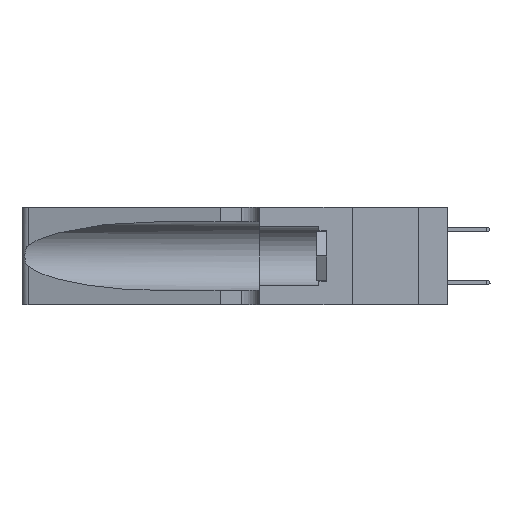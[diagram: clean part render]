
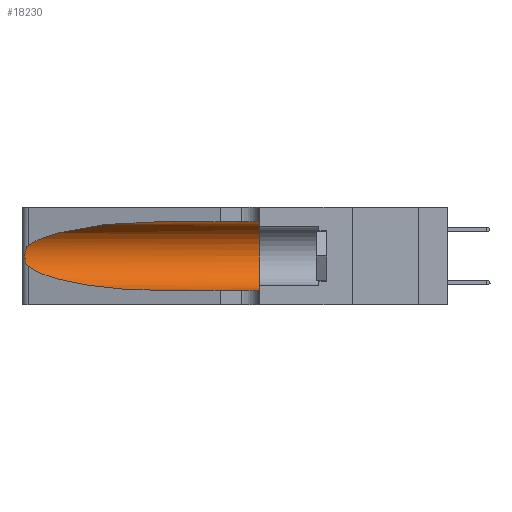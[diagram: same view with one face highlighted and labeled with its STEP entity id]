
A CAD part, left-side view. The second image highlights one B-rep face of the part: STEP entity #18230.
In plain terms, the highlighted cylindrical face has radius 3.308 mm (diameter 6.617 mm), a partial arc.
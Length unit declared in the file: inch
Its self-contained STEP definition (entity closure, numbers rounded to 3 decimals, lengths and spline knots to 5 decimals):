
#116 = CYLINDRICAL_SURFACE ( 'NONE', #184, 0.13025 ) ;
#184 = AXIS2_PLACEMENT_3D ( 'NONE', #6287, #4804, #3299 ) ;
#208 = ORIENTED_EDGE ( 'NONE', *, *, #14367, .T. ) ;
#456 = CARTESIAN_POINT ( 'NONE',  ( 0.25639, 1.23184, 0.21858 ) ) ;
#737 = VECTOR ( 'NONE', #8230, 39.37008 ) ;
#919 = DIRECTION ( 'NONE',  ( 0., -1., 0. ) ) ;
#948 = DIRECTION ( 'NONE',  ( 0., 0., 1. ) ) ;
#1972 = CARTESIAN_POINT ( 'NONE',  ( 0.25854, 1.2359, 0.20912 ) ) ;
#2413 = CARTESIAN_POINT ( 'NONE',  ( 0.1305, 0.72297, 0.31525 ) ) ;
#2427 = CARTESIAN_POINT ( 'NONE',  ( 0.1305, 1.61858, 0.05475 ) ) ;
#2509 =( BOUNDED_CURVE ( )  B_SPLINE_CURVE ( 3, ( #2413, #14236, #17169, #8345 ),
 .UNSPECIFIED., .F., .T. ) 
 B_SPLINE_CURVE_WITH_KNOTS ( ( 4, 4 ),
 ( 1.5708, 2.84003 ),
 .UNSPECIFIED. ) 
 CURVE ( )  GEOMETRIC_REPRESENTATION_ITEM ( )  RATIONAL_B_SPLINE_CURVE ( ( 1., 0.87, 0.87, 1. ) ) 
 REPRESENTATION_ITEM ( '' )  );
#2665 = VERTEX_POINT ( 'NONE', #16208 ) ;
#3154 = EDGE_CURVE ( 'NONE', #6895, #15905, #10402, .T. ) ;
#3299 = DIRECTION ( 'NONE',  ( 0., 0., -1. ) ) ;
#3495 = CARTESIAN_POINT ( 'NONE',  ( 0.26075, 1.23896, 0.19203 ) ) ;
#4143 = FACE_OUTER_BOUND ( 'NONE', #4858, .T. ) ;
#4450 = VERTEX_POINT ( 'NONE', #17107 ) ;
#4804 = DIRECTION ( 'NONE',  ( 0., -1., 0. ) ) ;
#4858 = EDGE_LOOP ( 'NONE', ( #208, #18872, #9476, #4998, #5190, #18024 ) ) ;
#4991 = CARTESIAN_POINT ( 'NONE',  ( 0.26017, 1.23833, 0.17102 ) ) ;
#4998 = ORIENTED_EDGE ( 'NONE', *, *, #18517, .T. ) ;
#5190 = ORIENTED_EDGE ( 'NONE', *, *, #16940, .F. ) ;
#5484 = CARTESIAN_POINT ( 'NONE',  ( 0.2373, 1.15595, 0.08982 ) ) ;
#5829 = CARTESIAN_POINT ( 'NONE',  ( 0.1305, 0.72297, 0.05475 ) ) ;
#6287 = CARTESIAN_POINT ( 'NONE',  ( 0.1305, 1.61858, 0.185 ) ) ;
#6468 = CARTESIAN_POINT ( 'NONE',  ( 0.25789, 1.23486, 0.15765 ) ) ;
#6856 = CARTESIAN_POINT ( 'NONE',  ( 0.25487, 1.22718, 0.14631 ) ) ;
#6864 = EDGE_CURVE ( 'NONE', #9983, #4450, #8609, .T. ) ;
#6874 = VECTOR ( 'NONE', #919, 39.37008 ) ;
#6895 = VERTEX_POINT ( 'NONE', #6856 ) ;
#7844 = CARTESIAN_POINT ( 'NONE',  ( 0.25487, 1.22718, 0.22369 ) ) ;
#7904 = CARTESIAN_POINT ( 'NONE',  ( 0.25555, 1.22993, 0.14849 ) ) ;
#8162 = CARTESIAN_POINT ( 'NONE',  ( 0.1305, 1.61858, 0.31525 ) ) ;
#8230 = DIRECTION ( 'NONE',  ( 0., -1., 0. ) ) ;
#8345 = CARTESIAN_POINT ( 'NONE',  ( 0.25487, 1.22718, 0.22369 ) ) ;
#8609 = LINE ( 'NONE', #8162, #737 ) ;
#9325 = CARTESIAN_POINT ( 'NONE',  ( 0.25555, 1.22994, 0.2215 ) ) ;
#9476 = ORIENTED_EDGE ( 'NONE', *, *, #3154, .T. ) ;
#9815 = DIRECTION ( 'NONE',  ( 0., 1., 0. ) ) ;
#9876 = CARTESIAN_POINT ( 'NONE',  ( 0.18966, 0.96281, 0.05475 ) ) ;
#9983 = VERTEX_POINT ( 'NONE', #12417 ) ;
#10402 =( BOUNDED_CURVE ( )  B_SPLINE_CURVE ( 3, ( #12870, #5484, #9876, #14346 ),
 .UNSPECIFIED., .F., .F. ) 
 B_SPLINE_CURVE_WITH_KNOTS ( ( 4, 4 ),
 ( 3.44316, 4.71239 ),
 .UNSPECIFIED. ) 
 CURVE ( )  GEOMETRIC_REPRESENTATION_ITEM ( )  RATIONAL_B_SPLINE_CURVE ( ( 1., 0.87, 0.87, 1. ) ) 
 REPRESENTATION_ITEM ( '' )  );
#10830 = CARTESIAN_POINT ( 'NONE',  ( 0.25787, 1.23484, 0.2124 ) ) ;
#11061 = CARTESIAN_POINT ( 'NONE',  ( 0.25487, 1.22718, 0.22369 ) ) ;
#11122 = EDGE_CURVE ( 'NONE', #11437, #6895, #16810, .T. ) ;
#11437 = VERTEX_POINT ( 'NONE', #11061 ) ;
#12302 = CARTESIAN_POINT ( 'NONE',  ( 0.26018, 1.23835, 0.19895 ) ) ;
#12417 = CARTESIAN_POINT ( 'NONE',  ( 0.1305, 0.72297, 0.31525 ) ) ;
#12870 = CARTESIAN_POINT ( 'NONE',  ( 0.25487, 1.22718, 0.14631 ) ) ;
#13787 = CARTESIAN_POINT ( 'NONE',  ( 0.26075, 1.23896, 0.178 ) ) ;
#14236 = CARTESIAN_POINT ( 'NONE',  ( 0.18966, 0.96281, 0.31525 ) ) ;
#14346 = CARTESIAN_POINT ( 'NONE',  ( 0.1305, 0.72297, 0.05475 ) ) ;
#14367 = EDGE_CURVE ( 'NONE', #9983, #11437, #2509, .T. ) ;
#15286 = CARTESIAN_POINT ( 'NONE',  ( 0.25856, 1.23593, 0.16098 ) ) ;
#15905 = VERTEX_POINT ( 'NONE', #5829 ) ;
#16208 = CARTESIAN_POINT ( 'NONE',  ( 0.1305, 0.35, 0.05475 ) ) ;
#16742 = CARTESIAN_POINT ( 'NONE',  ( 0.25639, 1.23186, 0.15144 ) ) ;
#16810 = B_SPLINE_CURVE_WITH_KNOTS ( 'NONE', 3,
 ( #7844, #9325, #456, #10830, #1972, #12302, #3495, #13787, #4991, #15286, #6468, #16742, #7904, #18205 ),
 .UNSPECIFIED., .F., .F.,
 ( 4, 2, 2, 2, 2, 2, 4 ),
 ( 0., 0.00027, 0.00053, 0.00107, 0.0016, 0.00187, 0.00214 ),
 .UNSPECIFIED. ) ;
#16895 = AXIS2_PLACEMENT_3D ( 'NONE', #18602, #9815, #948 ) ;
#16940 = EDGE_CURVE ( 'NONE', #4450, #2665, #18841, .T. ) ;
#17107 = CARTESIAN_POINT ( 'NONE',  ( 0.1305, 0.35, 0.31525 ) ) ;
#17169 = CARTESIAN_POINT ( 'NONE',  ( 0.2373, 1.15595, 0.28018 ) ) ;
#18024 = ORIENTED_EDGE ( 'NONE', *, *, #6864, .F. ) ;
#18205 = CARTESIAN_POINT ( 'NONE',  ( 0.25487, 1.22718, 0.14631 ) ) ;
#18230 = ADVANCED_FACE ( 'NONE', ( #4143 ), #116, .F. ) ;
#18517 = EDGE_CURVE ( 'NONE', #15905, #2665, #18566, .T. ) ;
#18566 = LINE ( 'NONE', #2427, #6874 ) ;
#18602 = CARTESIAN_POINT ( 'NONE',  ( 0.1305, 0.35, 0.185 ) ) ;
#18841 = CIRCLE ( 'NONE', #16895, 0.13025 ) ;
#18872 = ORIENTED_EDGE ( 'NONE', *, *, #11122, .T. ) ;
